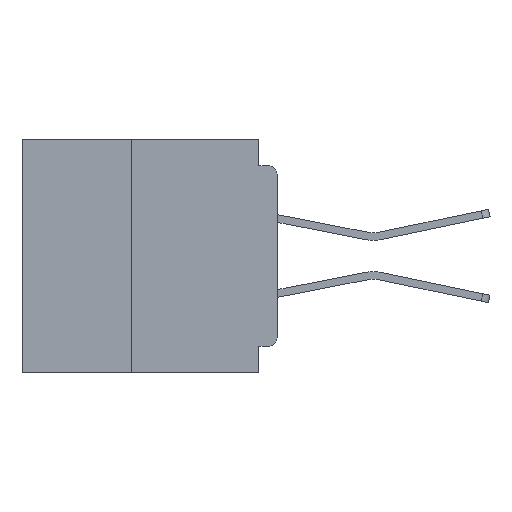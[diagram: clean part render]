
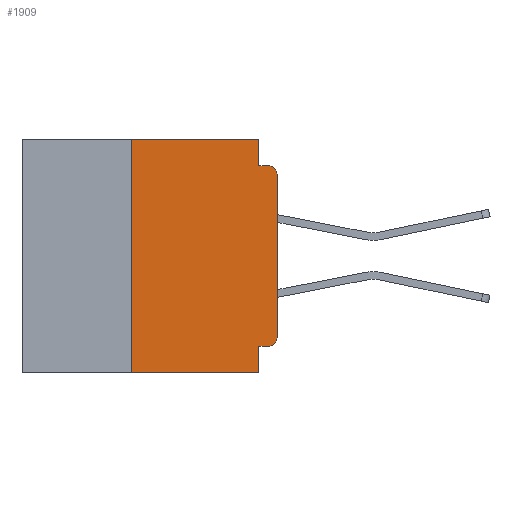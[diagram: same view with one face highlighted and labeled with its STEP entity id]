
A CAD part, left-side view. The second image highlights one B-rep face of the part: STEP entity #1909.
In plain terms, the highlighted planar face has unit normal (-1, 0, 0).
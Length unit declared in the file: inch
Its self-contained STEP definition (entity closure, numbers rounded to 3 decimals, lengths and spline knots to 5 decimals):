
#865 = LINE ( 'NONE', #19388, #16197 ) ;
#1193 = AXIS2_PLACEMENT_3D ( 'NONE', #39895, #2218, #38649 ) ;
#1330 = EDGE_CURVE ( 'NONE', #41574, #39042, #4798, .T. ) ;
#1909 = ADVANCED_FACE ( 'NONE', ( #16976 ), #9629, .F. ) ;
#2218 = DIRECTION ( 'NONE',  ( 1., 0., 0. ) ) ;
#2538 = ORIENTED_EDGE ( 'NONE', *, *, #1330, .F. ) ;
#2581 = ORIENTED_EDGE ( 'NONE', *, *, #33985, .T. ) ;
#2942 = LINE ( 'NONE', #14749, #20311 ) ;
#3294 = CARTESIAN_POINT ( 'NONE',  ( 0., 0., -0.355 ) ) ;
#3299 = CARTESIAN_POINT ( 'NONE',  ( 0., 0.25, -0.4 ) ) ;
#3336 = VERTEX_POINT ( 'NONE', #11064 ) ;
#3602 = CARTESIAN_POINT ( 'NONE',  ( 0., 0., 0. ) ) ;
#3800 = EDGE_CURVE ( 'NONE', #22530, #21715, #865, .T. ) ;
#3957 = DIRECTION ( 'NONE',  ( 0., 0., -1. ) ) ;
#4609 = ORIENTED_EDGE ( 'NONE', *, *, #3800, .F. ) ;
#4798 = LINE ( 'NONE', #7507, #29750 ) ;
#5604 = VERTEX_POINT ( 'NONE', #32991 ) ;
#6639 = DIRECTION ( 'NONE',  ( 0., 1., 0. ) ) ;
#7311 = CARTESIAN_POINT ( 'NONE',  ( 0., 0.031, -0.4 ) ) ;
#7464 = DIRECTION ( 'NONE',  ( 0., -1., 0. ) ) ;
#7507 = CARTESIAN_POINT ( 'NONE',  ( 0., 0., -0.045 ) ) ;
#8291 = ORIENTED_EDGE ( 'NONE', *, *, #9406, .F. ) ;
#9254 = ORIENTED_EDGE ( 'NONE', *, *, #27264, .T. ) ;
#9278 = CARTESIAN_POINT ( 'NONE',  ( 0., 0.031, 0. ) ) ;
#9305 = DIRECTION ( 'NONE',  ( -1., 0., 0. ) ) ;
#9406 = EDGE_CURVE ( 'NONE', #5604, #14665, #39968, .T. ) ;
#9629 = PLANE ( 'NONE',  #1193 ) ;
#10328 = EDGE_CURVE ( 'NONE', #21734, #34620, #14436, .T. ) ;
#10811 = ORIENTED_EDGE ( 'NONE', *, *, #38943, .F. ) ;
#11064 = CARTESIAN_POINT ( 'NONE',  ( 0., 0.015, -0.355 ) ) ;
#12824 = VECTOR ( 'NONE', #26068, 39.37008 ) ;
#13309 = CARTESIAN_POINT ( 'NONE',  ( 0., 0.015, -0.34 ) ) ;
#13843 = ORIENTED_EDGE ( 'NONE', *, *, #25836, .T. ) ;
#13958 = VECTOR ( 'NONE', #3957, 39.37008 ) ;
#14436 = LINE ( 'NONE', #3602, #21051 ) ;
#14665 = VERTEX_POINT ( 'NONE', #36482 ) ;
#14749 = CARTESIAN_POINT ( 'NONE',  ( 0., 0.437, -0.4 ) ) ;
#15987 = VECTOR ( 'NONE', #28827, 39.37008 ) ;
#16197 = VECTOR ( 'NONE', #18409, 39.37008 ) ;
#16560 = DIRECTION ( 'NONE',  ( 0., 0., -1. ) ) ;
#16839 = ORIENTED_EDGE ( 'NONE', *, *, #10328, .T. ) ;
#16976 = FACE_OUTER_BOUND ( 'NONE', #39696, .T. ) ;
#17105 = CARTESIAN_POINT ( 'NONE',  ( 0., 0.25, -0.4 ) ) ;
#18409 = DIRECTION ( 'NONE',  ( 0., -1., 0. ) ) ;
#19388 = CARTESIAN_POINT ( 'NONE',  ( 0., 0.437, 0. ) ) ;
#19888 = ORIENTED_EDGE ( 'NONE', *, *, #40551, .F. ) ;
#20311 = VECTOR ( 'NONE', #37555, 39.37008 ) ;
#20457 = VECTOR ( 'NONE', #6639, 39.37008 ) ;
#20945 = CARTESIAN_POINT ( 'NONE',  ( 0., 0.031, -0.045 ) ) ;
#20968 = CARTESIAN_POINT ( 'NONE',  ( 0., 0.25, 0. ) ) ;
#21051 = VECTOR ( 'NONE', #23094, 39.37008 ) ;
#21715 = VERTEX_POINT ( 'NONE', #34378 ) ;
#21734 = VERTEX_POINT ( 'NONE', #24672 ) ;
#22530 = VERTEX_POINT ( 'NONE', #20968 ) ;
#23094 = DIRECTION ( 'NONE',  ( 0., 0., 1. ) ) ;
#24601 = LINE ( 'NONE', #9278, #15987 ) ;
#24672 = CARTESIAN_POINT ( 'NONE',  ( 0., 0., -0.34 ) ) ;
#25734 = CIRCLE ( 'NONE', #42183, 0.015 ) ;
#25836 = EDGE_CURVE ( 'NONE', #28419, #14665, #2942, .T. ) ;
#26068 = DIRECTION ( 'NONE',  ( 0., 0., 1. ) ) ;
#27264 = EDGE_CURVE ( 'NONE', #34620, #39042, #25734, .T. ) ;
#28419 = VERTEX_POINT ( 'NONE', #17105 ) ;
#28726 = CARTESIAN_POINT ( 'NONE',  ( 0., 0.015, -0.06 ) ) ;
#28827 = DIRECTION ( 'NONE',  ( 0., 0., -1. ) ) ;
#29750 = VECTOR ( 'NONE', #7464, 39.37008 ) ;
#30043 = EDGE_CURVE ( 'NONE', #3336, #5604, #30136, .T. ) ;
#30136 = LINE ( 'NONE', #3294, #20457 ) ;
#32006 = DIRECTION ( 'NONE',  ( 0., 0., -1. ) ) ;
#32009 = CIRCLE ( 'NONE', #37089, 0.015 ) ;
#32991 = CARTESIAN_POINT ( 'NONE',  ( 0., 0.031, -0.355 ) ) ;
#33985 = EDGE_CURVE ( 'NONE', #3336, #21734, #32009, .T. ) ;
#34172 = ORIENTED_EDGE ( 'NONE', *, *, #30043, .F. ) ;
#34378 = CARTESIAN_POINT ( 'NONE',  ( 0., 0.031, 0. ) ) ;
#34507 = CARTESIAN_POINT ( 'NONE',  ( 0., 0.015, -0.045 ) ) ;
#34620 = VERTEX_POINT ( 'NONE', #35756 ) ;
#35756 = CARTESIAN_POINT ( 'NONE',  ( 0., 0., -0.06 ) ) ;
#36089 = DIRECTION ( 'NONE',  ( -1., 0., 0. ) ) ;
#36482 = CARTESIAN_POINT ( 'NONE',  ( 0., 0.031, -0.4 ) ) ;
#37089 = AXIS2_PLACEMENT_3D ( 'NONE', #13309, #36089, #16560 ) ;
#37555 = DIRECTION ( 'NONE',  ( 0., -1., 0. ) ) ;
#37774 = LINE ( 'NONE', #3299, #12824 ) ;
#38649 = DIRECTION ( 'NONE',  ( 0., 0., -1. ) ) ;
#38943 = EDGE_CURVE ( 'NONE', #28419, #22530, #37774, .T. ) ;
#39042 = VERTEX_POINT ( 'NONE', #34507 ) ;
#39696 = EDGE_LOOP ( 'NONE', ( #16839, #9254, #2538, #19888, #4609, #10811, #13843, #8291, #34172, #2581 ) ) ;
#39895 = CARTESIAN_POINT ( 'NONE',  ( 0., 0.437, 0. ) ) ;
#39968 = LINE ( 'NONE', #7311, #13958 ) ;
#40551 = EDGE_CURVE ( 'NONE', #21715, #41574, #24601, .T. ) ;
#41574 = VERTEX_POINT ( 'NONE', #20945 ) ;
#42183 = AXIS2_PLACEMENT_3D ( 'NONE', #28726, #9305, #32006 ) ;
